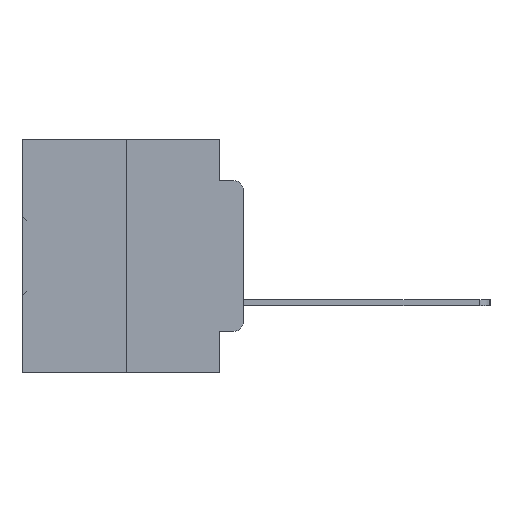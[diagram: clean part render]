
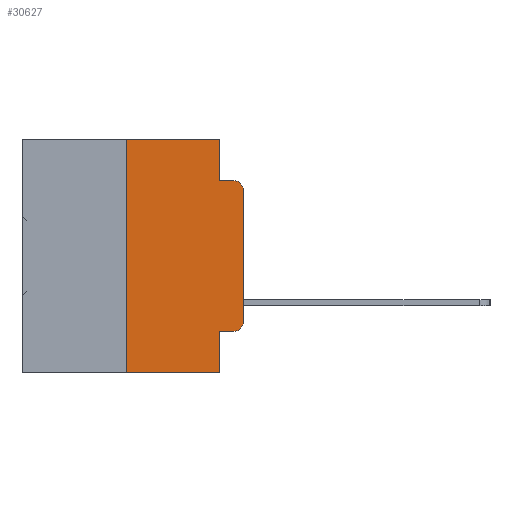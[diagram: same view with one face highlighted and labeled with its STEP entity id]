
A CAD part, left-side view. The second image highlights one B-rep face of the part: STEP entity #30627.
In plain terms, the highlighted planar face has unit normal (-1, 0, 0).
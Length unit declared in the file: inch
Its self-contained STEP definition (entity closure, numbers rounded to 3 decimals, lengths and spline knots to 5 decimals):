
#796 = DIRECTION ( 'NONE',  ( 0., -1., 0. ) ) ;
#1027 = CARTESIAN_POINT ( 'NONE',  ( 0., 0.02, -0.0885 ) ) ;
#1429 = CARTESIAN_POINT ( 'NONE',  ( 0., 0.02, -0.3915 ) ) ;
#3982 = CARTESIAN_POINT ( 'NONE',  ( 0., 0.25, 0. ) ) ;
#4406 = CARTESIAN_POINT ( 'NONE',  ( 0., 0., -0.3915 ) ) ;
#4477 = DIRECTION ( 'NONE',  ( 0., 0., -1. ) ) ;
#4875 = ORIENTED_EDGE ( 'NONE', *, *, #14329, .F. ) ;
#5304 = DIRECTION ( 'NONE',  ( 0., 0., 1. ) ) ;
#5412 = ORIENTED_EDGE ( 'NONE', *, *, #28232, .T. ) ;
#5671 = FACE_OUTER_BOUND ( 'NONE', #6494, .T. ) ;
#5824 = VERTEX_POINT ( 'NONE', #35183 ) ;
#6477 = VECTOR ( 'NONE', #796, 39.37008 ) ;
#6494 = EDGE_LOOP ( 'NONE', ( #17875, #27201, #4875, #6764, #26338, #20170, #29458, #9509, #5412, #25035 ) ) ;
#6561 = CARTESIAN_POINT ( 'NONE',  ( 0., 0.051, 0. ) ) ;
#6764 = ORIENTED_EDGE ( 'NONE', *, *, #12647, .F. ) ;
#7569 = VERTEX_POINT ( 'NONE', #15209 ) ;
#7629 = VERTEX_POINT ( 'NONE', #1027 ) ;
#8857 = CARTESIAN_POINT ( 'NONE',  ( 0., 0.051, -0.0885 ) ) ;
#9190 = VECTOR ( 'NONE', #36986, 39.37008 ) ;
#9509 = ORIENTED_EDGE ( 'NONE', *, *, #19436, .F. ) ;
#9522 = LINE ( 'NONE', #8857, #16169 ) ;
#11083 = VERTEX_POINT ( 'NONE', #28167 ) ;
#12082 = VECTOR ( 'NONE', #29427, 39.37008 ) ;
#12194 = CARTESIAN_POINT ( 'NONE',  ( 0., 0., -0.1085 ) ) ;
#12320 = DIRECTION ( 'NONE',  ( 0., 0., -1. ) ) ;
#12647 = EDGE_CURVE ( 'NONE', #7569, #20030, #16308, .T. ) ;
#12695 = VECTOR ( 'NONE', #30274, 39.37008 ) ;
#12730 = DIRECTION ( 'NONE',  ( 1., 0., 0. ) ) ;
#13204 = AXIS2_PLACEMENT_3D ( 'NONE', #35263, #12730, #32555 ) ;
#13713 = CARTESIAN_POINT ( 'NONE',  ( 0., 0.25, -0.5 ) ) ;
#13783 = VECTOR ( 'NONE', #18938, 39.37008 ) ;
#14140 = VERTEX_POINT ( 'NONE', #13713 ) ;
#14167 = LINE ( 'NONE', #22159, #28365 ) ;
#14329 = EDGE_CURVE ( 'NONE', #20030, #7629, #9522, .T. ) ;
#14756 = DIRECTION ( 'NONE',  ( -1., 0., 0. ) ) ;
#15209 = CARTESIAN_POINT ( 'NONE',  ( 0., 0.051, 0. ) ) ;
#15835 = LINE ( 'NONE', #25734, #9190 ) ;
#16083 = CARTESIAN_POINT ( 'NONE',  ( 0., 0.051, -0.4115 ) ) ;
#16169 = VECTOR ( 'NONE', #31546, 39.37008 ) ;
#16209 = VERTEX_POINT ( 'NONE', #4406 ) ;
#16308 = LINE ( 'NONE', #6561, #37123 ) ;
#17875 = ORIENTED_EDGE ( 'NONE', *, *, #30184, .T. ) ;
#18458 = CARTESIAN_POINT ( 'NONE',  ( 0., 0.051, -0.0885 ) ) ;
#18629 = AXIS2_PLACEMENT_3D ( 'NONE', #31742, #14756, #34567 ) ;
#18938 = DIRECTION ( 'NONE',  ( 0., -1., 0. ) ) ;
#19436 = EDGE_CURVE ( 'NONE', #20451, #5824, #35282, .T. ) ;
#19760 = EDGE_CURVE ( 'NONE', #29085, #7629, #31301, .T. ) ;
#20030 = VERTEX_POINT ( 'NONE', #18458 ) ;
#20170 = ORIENTED_EDGE ( 'NONE', *, *, #23915, .F. ) ;
#20451 = VERTEX_POINT ( 'NONE', #29098 ) ;
#20693 = EDGE_CURVE ( 'NONE', #11083, #16209, #22797, .T. ) ;
#21626 = DIRECTION ( 'NONE',  ( -1., 0., 0. ) ) ;
#22159 = CARTESIAN_POINT ( 'NONE',  ( 0., 0.25, 0. ) ) ;
#22797 = CIRCLE ( 'NONE', #24107, 0.02 ) ;
#23618 = VERTEX_POINT ( 'NONE', #3982 ) ;
#23915 = EDGE_CURVE ( 'NONE', #14140, #23618, #14167, .T. ) ;
#24107 = AXIS2_PLACEMENT_3D ( 'NONE', #1429, #21626, #4477 ) ;
#25035 = ORIENTED_EDGE ( 'NONE', *, *, #20693, .T. ) ;
#25734 = CARTESIAN_POINT ( 'NONE',  ( 0., 0., 0. ) ) ;
#26338 = ORIENTED_EDGE ( 'NONE', *, *, #30238, .F. ) ;
#27201 = ORIENTED_EDGE ( 'NONE', *, *, #19760, .T. ) ;
#28167 = CARTESIAN_POINT ( 'NONE',  ( 0., 0.02, -0.4115 ) ) ;
#28232 = EDGE_CURVE ( 'NONE', #20451, #11083, #36358, .T. ) ;
#28365 = VECTOR ( 'NONE', #5304, 39.37008 ) ;
#29085 = VERTEX_POINT ( 'NONE', #12194 ) ;
#29098 = CARTESIAN_POINT ( 'NONE',  ( 0., 0.051, -0.4115 ) ) ;
#29158 = LINE ( 'NONE', #34394, #6477 ) ;
#29427 = DIRECTION ( 'NONE',  ( 0., -1., 0. ) ) ;
#29458 = ORIENTED_EDGE ( 'NONE', *, *, #34996, .T. ) ;
#29712 = PLANE ( 'NONE',  #13204 ) ;
#30184 = EDGE_CURVE ( 'NONE', #16209, #29085, #15835, .T. ) ;
#30238 = EDGE_CURVE ( 'NONE', #23618, #7569, #29158, .T. ) ;
#30274 = DIRECTION ( 'NONE',  ( 0., 0., -1. ) ) ;
#30627 = ADVANCED_FACE ( 'NONE', ( #5671 ), #29712, .F. ) ;
#31301 = CIRCLE ( 'NONE', #18629, 0.02 ) ;
#31546 = DIRECTION ( 'NONE',  ( 0., -1., 0. ) ) ;
#31742 = CARTESIAN_POINT ( 'NONE',  ( 0., 0.02, -0.1085 ) ) ;
#32555 = DIRECTION ( 'NONE',  ( 0., 0., -1. ) ) ;
#32985 = CARTESIAN_POINT ( 'NONE',  ( 0., 0.051, 0. ) ) ;
#33781 = LINE ( 'NONE', #35099, #12082 ) ;
#34394 = CARTESIAN_POINT ( 'NONE',  ( 0., 0.473, 0. ) ) ;
#34567 = DIRECTION ( 'NONE',  ( 0., 0., -1. ) ) ;
#34996 = EDGE_CURVE ( 'NONE', #14140, #5824, #33781, .T. ) ;
#35099 = CARTESIAN_POINT ( 'NONE',  ( 0., 0.473, -0.5 ) ) ;
#35183 = CARTESIAN_POINT ( 'NONE',  ( 0., 0.051, -0.5 ) ) ;
#35263 = CARTESIAN_POINT ( 'NONE',  ( 0., 0.473, 0. ) ) ;
#35282 = LINE ( 'NONE', #32985, #12695 ) ;
#36358 = LINE ( 'NONE', #16083, #13783 ) ;
#36986 = DIRECTION ( 'NONE',  ( 0., 0., 1. ) ) ;
#37123 = VECTOR ( 'NONE', #12320, 39.37008 ) ;
